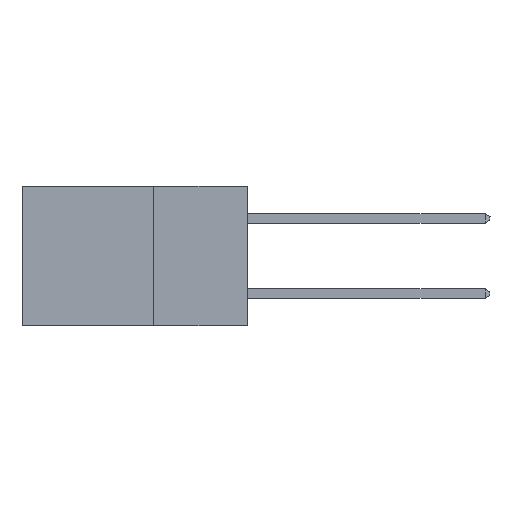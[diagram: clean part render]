
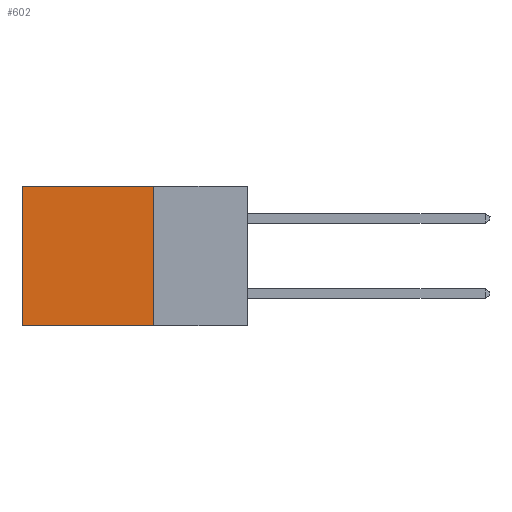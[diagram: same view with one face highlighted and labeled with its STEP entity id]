
A CAD part, left-side view. The second image highlights one B-rep face of the part: STEP entity #602.
In plain terms, the highlighted planar face has unit normal (-1, 0, 0).
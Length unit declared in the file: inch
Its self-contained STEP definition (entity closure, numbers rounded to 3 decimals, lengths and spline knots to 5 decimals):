
#250 = AXIS2_PLACEMENT_3D ( 'NONE', #7332, #9296, #8311 ) ;
#602 = ADVANCED_FACE ( 'NONE', ( #10321 ), #8518, .F. ) ;
#616 = EDGE_CURVE ( 'NONE', #8110, #1176, #12545, .T. ) ;
#1176 = VERTEX_POINT ( 'NONE', #9830 ) ;
#1708 = ORIENTED_EDGE ( 'NONE', *, *, #13068, .T. ) ;
#2196 = VERTEX_POINT ( 'NONE', #8474 ) ;
#2857 = VECTOR ( 'NONE', #4321, 39.37008 ) ;
#3077 = VERTEX_POINT ( 'NONE', #10563 ) ;
#3337 = DIRECTION ( 'NONE',  ( 0., 1., 0. ) ) ;
#3463 = CARTESIAN_POINT ( 'NONE',  ( 0.2615, 0.25, 0. ) ) ;
#4321 = DIRECTION ( 'NONE',  ( 0., 1., 0. ) ) ;
#4415 = EDGE_CURVE ( 'NONE', #2196, #8110, #12936, .T. ) ;
#5082 = LINE ( 'NONE', #12114, #8003 ) ;
#5905 = DIRECTION ( 'NONE',  ( 0., 0., -1. ) ) ;
#6316 = LINE ( 'NONE', #3463, #2857 ) ;
#6542 = ORIENTED_EDGE ( 'NONE', *, *, #616, .F. ) ;
#6904 = CARTESIAN_POINT ( 'NONE',  ( 0.2615, 0.25, -0.37 ) ) ;
#7332 = CARTESIAN_POINT ( 'NONE',  ( 0.2615, 0.25, -0.37 ) ) ;
#8003 = VECTOR ( 'NONE', #11235, 39.37008 ) ;
#8110 = VERTEX_POINT ( 'NONE', #9601 ) ;
#8311 = DIRECTION ( 'NONE',  ( 0., 0., -1. ) ) ;
#8409 = ORIENTED_EDGE ( 'NONE', *, *, #4415, .F. ) ;
#8474 = CARTESIAN_POINT ( 'NONE',  ( 0.2615, 0.25, 0. ) ) ;
#8518 = PLANE ( 'NONE',  #250 ) ;
#9296 = DIRECTION ( 'NONE',  ( 1., 0., 0. ) ) ;
#9601 = CARTESIAN_POINT ( 'NONE',  ( 0.2615, 0.25, -0.37 ) ) ;
#9830 = CARTESIAN_POINT ( 'NONE',  ( 0.2615, 0.6, -0.37 ) ) ;
#9856 = VECTOR ( 'NONE', #5905, 39.37008 ) ;
#10321 = FACE_OUTER_BOUND ( 'NONE', #11740, .T. ) ;
#10389 = CARTESIAN_POINT ( 'NONE',  ( 0.2615, 0.25, -0.37 ) ) ;
#10563 = CARTESIAN_POINT ( 'NONE',  ( 0.2615, 0.6, 0. ) ) ;
#10845 = EDGE_CURVE ( 'NONE', #2196, #3077, #6316, .T. ) ;
#11235 = DIRECTION ( 'NONE',  ( 0., 0., -1. ) ) ;
#11321 = VECTOR ( 'NONE', #3337, 39.37008 ) ;
#11740 = EDGE_LOOP ( 'NONE', ( #1708, #6542, #8409, #13114 ) ) ;
#12114 = CARTESIAN_POINT ( 'NONE',  ( 0.2615, 0.6, -0.37 ) ) ;
#12545 = LINE ( 'NONE', #10389, #11321 ) ;
#12936 = LINE ( 'NONE', #6904, #9856 ) ;
#13068 = EDGE_CURVE ( 'NONE', #3077, #1176, #5082, .T. ) ;
#13114 = ORIENTED_EDGE ( 'NONE', *, *, #10845, .T. ) ;
